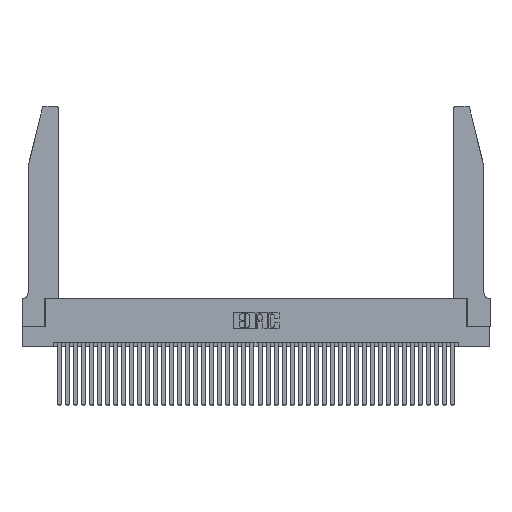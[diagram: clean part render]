
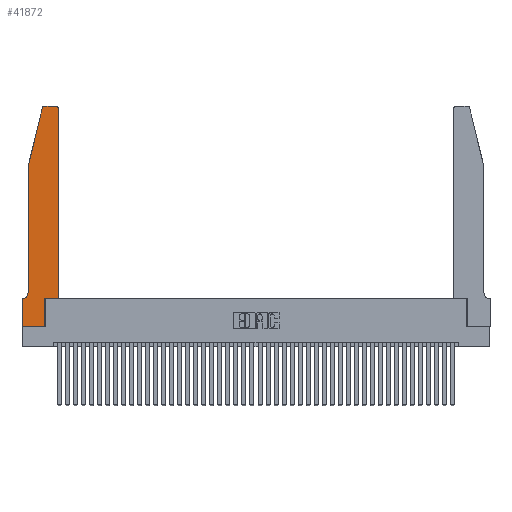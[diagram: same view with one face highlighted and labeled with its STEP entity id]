
A CAD part, top view. The second image highlights one B-rep face of the part: STEP entity #41872.
In plain terms, the highlighted planar face has unit normal (0, 0, 1).
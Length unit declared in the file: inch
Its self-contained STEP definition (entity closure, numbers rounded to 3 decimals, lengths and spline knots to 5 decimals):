
#24 = VERTEX_POINT ( 'NONE', #36834 ) ;
#1010 = CIRCLE ( 'NONE', #32408, 0.03 ) ;
#1539 = EDGE_CURVE ( 'NONE', #38981, #38687, #4493, .T. ) ;
#1946 = CARTESIAN_POINT ( 'NONE',  ( 0.0055, 0.35, 0.37 ) ) ;
#2404 = ORIENTED_EDGE ( 'NONE', *, *, #10834, .T. ) ;
#2922 = LINE ( 'NONE', #11637, #36008 ) ;
#3956 = FACE_OUTER_BOUND ( 'NONE', #18568, .T. ) ;
#4493 = LINE ( 'NONE', #22444, #11241 ) ;
#4660 = DIRECTION ( 'NONE',  ( 0., 0., 1. ) ) ;
#4727 = CARTESIAN_POINT ( 'NONE',  ( 0., 0.35, 0.37 ) ) ;
#5616 = EDGE_CURVE ( 'NONE', #12208, #13765, #1010, .T. ) ;
#6294 = VECTOR ( 'NONE', #39660, 39.37008 ) ;
#6629 = ORIENTED_EDGE ( 'NONE', *, *, #10088, .T. ) ;
#6648 = EDGE_CURVE ( 'NONE', #32325, #13306, #30456, .T. ) ;
#7336 = VECTOR ( 'NONE', #26426, 39.37008 ) ;
#8101 = DIRECTION ( 'NONE',  ( 1., 0., 0. ) ) ;
#9735 = ORIENTED_EDGE ( 'NONE', *, *, #17234, .T. ) ;
#10088 = EDGE_CURVE ( 'NONE', #13306, #27929, #32279, .T. ) ;
#10329 = CARTESIAN_POINT ( 'NONE',  ( 0., 0., 0.37 ) ) ;
#10383 = AXIS2_PLACEMENT_3D ( 'NONE', #24545, #4660, #27835 ) ;
#10834 = EDGE_CURVE ( 'NONE', #11791, #34099, #37276, .T. ) ;
#11241 = VECTOR ( 'NONE', #42140, 39.37008 ) ;
#11346 = VERTEX_POINT ( 'NONE', #36633 ) ;
#11633 = EDGE_CURVE ( 'NONE', #13765, #11791, #33703, .T. ) ;
#11637 = CARTESIAN_POINT ( 'NONE',  ( 0.2865, 0.35, 0.37 ) ) ;
#11656 = EDGE_CURVE ( 'NONE', #38687, #12208, #15083, .T. ) ;
#11791 = VERTEX_POINT ( 'NONE', #17864 ) ;
#12208 = VERTEX_POINT ( 'NONE', #39350 ) ;
#12457 = DIRECTION ( 'NONE',  ( 0., -1., 0. ) ) ;
#12845 = ORIENTED_EDGE ( 'NONE', *, *, #11656, .T. ) ;
#13306 = VERTEX_POINT ( 'NONE', #37983 ) ;
#13343 = ORIENTED_EDGE ( 'NONE', *, *, #39011, .T. ) ;
#13653 = DIRECTION ( 'NONE',  ( 1., 0., 0. ) ) ;
#13685 = EDGE_CURVE ( 'NONE', #24, #11346, #29190, .T. ) ;
#13765 = VERTEX_POINT ( 'NONE', #23955 ) ;
#13770 = CARTESIAN_POINT ( 'NONE',  ( 0.4205, 2.72, 0.37 ) ) ;
#14144 = DIRECTION ( 'NONE',  ( 0., 0., -1. ) ) ;
#14952 = DIRECTION ( 'NONE',  ( 0., 1., 0. ) ) ;
#15083 = LINE ( 'NONE', #16710, #6294 ) ;
#16457 = ORIENTED_EDGE ( 'NONE', *, *, #40565, .T. ) ;
#16614 = LINE ( 'NONE', #17462, #41777 ) ;
#16710 = CARTESIAN_POINT ( 'NONE',  ( 0.4505, 0.35, 0.37 ) ) ;
#17095 = DIRECTION ( 'NONE',  ( 1., 0., 0. ) ) ;
#17234 = EDGE_CURVE ( 'NONE', #11346, #38981, #2922, .T. ) ;
#17321 = CARTESIAN_POINT ( 'NONE',  ( 0.2865, 0.35, 0.37 ) ) ;
#17462 = CARTESIAN_POINT ( 'NONE',  ( 0.0755, 2., 0.37 ) ) ;
#17864 = CARTESIAN_POINT ( 'NONE',  ( 0.284, 2.75, 0.37 ) ) ;
#18568 = EDGE_LOOP ( 'NONE', ( #19083, #2404, #13343, #30931, #6629, #32991, #16457, #26333, #9735, #29403, #12845, #30430 ) ) ;
#19083 = ORIENTED_EDGE ( 'NONE', *, *, #11633, .T. ) ;
#19299 = CARTESIAN_POINT ( 'NONE',  ( 0.4505, 0.35, 0.37 ) ) ;
#20712 = AXIS2_PLACEMENT_3D ( 'NONE', #4727, #27897, #8101 ) ;
#20859 = DIRECTION ( 'NONE',  ( -0.239, -0.971, 0. ) ) ;
#21479 = VECTOR ( 'NONE', #13653, 39.37008 ) ;
#22444 = CARTESIAN_POINT ( 'NONE',  ( 0.4505, 0.35, 0.37 ) ) ;
#23108 = CARTESIAN_POINT ( 'NONE',  ( 0.2605, 2.75, 0.37 ) ) ;
#23302 = VECTOR ( 'NONE', #12457, 39.37008 ) ;
#23909 = VERTEX_POINT ( 'NONE', #31402 ) ;
#23955 = CARTESIAN_POINT ( 'NONE',  ( 0.4205, 2.75, 0.37 ) ) ;
#24227 = VECTOR ( 'NONE', #25822, 39.37008 ) ;
#24545 = CARTESIAN_POINT ( 'NONE',  ( 0.284, 2.72, 0.37 ) ) ;
#24615 = PLANE ( 'NONE',  #20712 ) ;
#25822 = DIRECTION ( 'NONE',  ( -1., 0., 0. ) ) ;
#26333 = ORIENTED_EDGE ( 'NONE', *, *, #13685, .T. ) ;
#26426 = DIRECTION ( 'NONE',  ( -1., 0., 0. ) ) ;
#27364 = VECTOR ( 'NONE', #38134, 39.37008 ) ;
#27835 = DIRECTION ( 'NONE',  ( 1., 0., 0. ) ) ;
#27897 = DIRECTION ( 'NONE',  ( 0., 0., 1. ) ) ;
#27929 = VERTEX_POINT ( 'NONE', #1946 ) ;
#28163 = CARTESIAN_POINT ( 'NONE',  ( 0.0755, 2., 0.37 ) ) ;
#28385 = AXIS2_PLACEMENT_3D ( 'NONE', #33935, #14144, #37147 ) ;
#28953 = CARTESIAN_POINT ( 'NONE',  ( 0., 0., 0.37 ) ) ;
#29190 = LINE ( 'NONE', #10329, #21479 ) ;
#29403 = ORIENTED_EDGE ( 'NONE', *, *, #1539, .T. ) ;
#30430 = ORIENTED_EDGE ( 'NONE', *, *, #5616, .T. ) ;
#30456 = LINE ( 'NONE', #31758, #27364 ) ;
#30931 = ORIENTED_EDGE ( 'NONE', *, *, #6648, .T. ) ;
#31402 = CARTESIAN_POINT ( 'NONE',  ( 0., 0.35, 0.37 ) ) ;
#31758 = CARTESIAN_POINT ( 'NONE',  ( 0.0755, 2., 0.37 ) ) ;
#32279 = CIRCLE ( 'NONE', #28385, 0.07 ) ;
#32325 = VERTEX_POINT ( 'NONE', #28163 ) ;
#32408 = AXIS2_PLACEMENT_3D ( 'NONE', #13770, #36781, #17095 ) ;
#32972 = LINE ( 'NONE', #35531, #24227 ) ;
#32991 = ORIENTED_EDGE ( 'NONE', *, *, #33065, .T. ) ;
#33065 = EDGE_CURVE ( 'NONE', #27929, #23909, #32972, .T. ) ;
#33703 = LINE ( 'NONE', #23108, #7336 ) ;
#33935 = CARTESIAN_POINT ( 'NONE',  ( 0.0055, 0.42, 0.37 ) ) ;
#34099 = VERTEX_POINT ( 'NONE', #34474 ) ;
#34474 = CARTESIAN_POINT ( 'NONE',  ( 0.25487, 2.72718, 0.37 ) ) ;
#35531 = CARTESIAN_POINT ( 'NONE',  ( 0.0755, 0.35, 0.37 ) ) ;
#36008 = VECTOR ( 'NONE', #14952, 39.37008 ) ;
#36633 = CARTESIAN_POINT ( 'NONE',  ( 0.2865, 0., 0.37 ) ) ;
#36781 = DIRECTION ( 'NONE',  ( 0., 0., 1. ) ) ;
#36834 = CARTESIAN_POINT ( 'NONE',  ( 0., 0., 0.37 ) ) ;
#37147 = DIRECTION ( 'NONE',  ( -1., 0., 0. ) ) ;
#37276 = CIRCLE ( 'NONE', #10383, 0.03 ) ;
#37983 = CARTESIAN_POINT ( 'NONE',  ( 0.0755, 0.42, 0.37 ) ) ;
#38134 = DIRECTION ( 'NONE',  ( 0., -1., 0. ) ) ;
#38687 = VERTEX_POINT ( 'NONE', #19299 ) ;
#38981 = VERTEX_POINT ( 'NONE', #17321 ) ;
#39011 = EDGE_CURVE ( 'NONE', #34099, #32325, #16614, .T. ) ;
#39350 = CARTESIAN_POINT ( 'NONE',  ( 0.4505, 2.72, 0.37 ) ) ;
#39660 = DIRECTION ( 'NONE',  ( 0., 1., 0. ) ) ;
#40565 = EDGE_CURVE ( 'NONE', #23909, #24, #41700, .T. ) ;
#41700 = LINE ( 'NONE', #28953, #23302 ) ;
#41777 = VECTOR ( 'NONE', #20859, 39.37008 ) ;
#41872 = ADVANCED_FACE ( 'NONE', ( #3956 ), #24615, .T. ) ;
#42140 = DIRECTION ( 'NONE',  ( 1., 0., 0. ) ) ;
